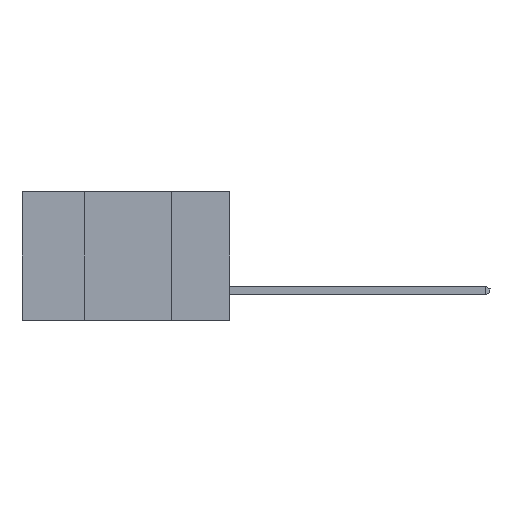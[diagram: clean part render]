
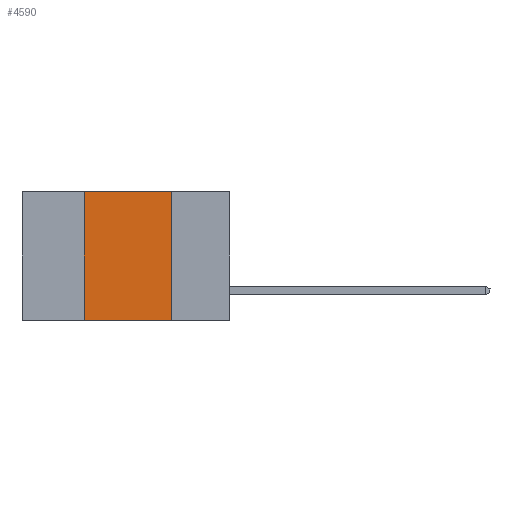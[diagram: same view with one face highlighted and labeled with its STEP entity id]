
A CAD part, left-side view. The second image highlights one B-rep face of the part: STEP entity #4590.
In plain terms, the highlighted planar face has unit normal (-1, 0, 0).
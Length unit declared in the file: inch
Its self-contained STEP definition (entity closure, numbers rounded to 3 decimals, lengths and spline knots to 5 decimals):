
#133 = LINE ( 'NONE', #15856, #17265 ) ;
#779 = EDGE_LOOP ( 'NONE', ( #16925, #2390, #16577, #11141 ) ) ;
#933 = CARTESIAN_POINT ( 'NONE',  ( 0., 0.6, -0.37 ) ) ;
#2390 = ORIENTED_EDGE ( 'NONE', *, *, #9555, .F. ) ;
#3868 = CARTESIAN_POINT ( 'NONE',  ( 0., 0.6, 0. ) ) ;
#4098 = CARTESIAN_POINT ( 'NONE',  ( 0., 0.42, -0.37 ) ) ;
#4156 = CARTESIAN_POINT ( 'NONE',  ( 0., 0.6, 0. ) ) ;
#4590 = ADVANCED_FACE ( 'NONE', ( #7058 ), #5733, .F. ) ;
#5306 = VECTOR ( 'NONE', #6491, 39.37008 ) ;
#5517 = EDGE_CURVE ( 'NONE', #12143, #6295, #133, .T. ) ;
#5733 = PLANE ( 'NONE',  #7922 ) ;
#6295 = VERTEX_POINT ( 'NONE', #14132 ) ;
#6491 = DIRECTION ( 'NONE',  ( 0., -1., 0. ) ) ;
#7058 = FACE_OUTER_BOUND ( 'NONE', #779, .T. ) ;
#7251 = DIRECTION ( 'NONE',  ( 1., 0., 0. ) ) ;
#7922 = AXIS2_PLACEMENT_3D ( 'NONE', #4156, #7251, #13038 ) ;
#8074 = LINE ( 'NONE', #18513, #12455 ) ;
#9555 = EDGE_CURVE ( 'NONE', #17772, #12143, #16860, .T. ) ;
#9941 = EDGE_CURVE ( 'NONE', #14113, #6295, #15338, .T. ) ;
#11141 = ORIENTED_EDGE ( 'NONE', *, *, #9941, .T. ) ;
#11261 = EDGE_CURVE ( 'NONE', #14113, #17772, #8074, .T. ) ;
#11735 = DIRECTION ( 'NONE',  ( 0., 0., -1. ) ) ;
#12143 = VERTEX_POINT ( 'NONE', #14302 ) ;
#12455 = VECTOR ( 'NONE', #12694, 39.37008 ) ;
#12694 = DIRECTION ( 'NONE',  ( 0., 0., 1. ) ) ;
#13038 = DIRECTION ( 'NONE',  ( 0., 0., -1. ) ) ;
#13938 = DIRECTION ( 'NONE',  ( 0., -1., 0. ) ) ;
#14113 = VERTEX_POINT ( 'NONE', #4098 ) ;
#14132 = CARTESIAN_POINT ( 'NONE',  ( 0., 0.17, -0.37 ) ) ;
#14302 = CARTESIAN_POINT ( 'NONE',  ( 0., 0.17, 0. ) ) ;
#15338 = LINE ( 'NONE', #933, #18505 ) ;
#15856 = CARTESIAN_POINT ( 'NONE',  ( 0., 0.17, -0.37 ) ) ;
#16076 = CARTESIAN_POINT ( 'NONE',  ( 0., 0.42, 0. ) ) ;
#16577 = ORIENTED_EDGE ( 'NONE', *, *, #11261, .F. ) ;
#16860 = LINE ( 'NONE', #3868, #5306 ) ;
#16925 = ORIENTED_EDGE ( 'NONE', *, *, #5517, .F. ) ;
#17265 = VECTOR ( 'NONE', #11735, 39.37008 ) ;
#17772 = VERTEX_POINT ( 'NONE', #16076 ) ;
#18505 = VECTOR ( 'NONE', #13938, 39.37008 ) ;
#18513 = CARTESIAN_POINT ( 'NONE',  ( 0., 0.42, -0.37 ) ) ;
